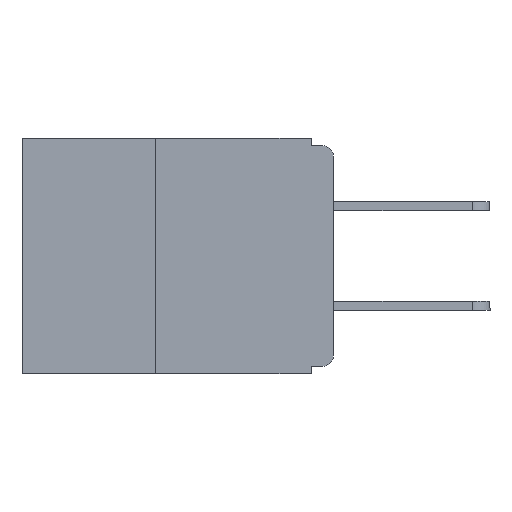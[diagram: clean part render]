
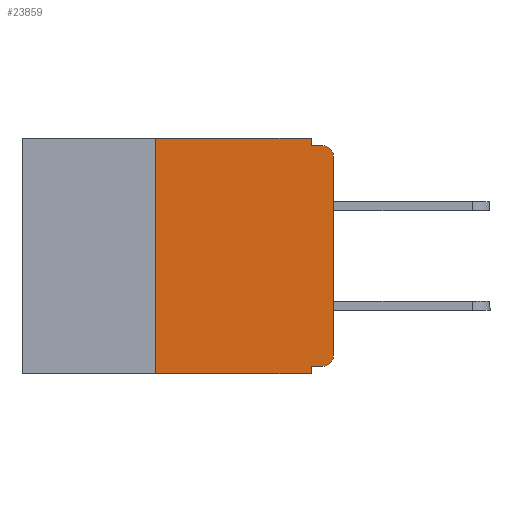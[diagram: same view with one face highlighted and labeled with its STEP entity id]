
A CAD part, left-side view. The second image highlights one B-rep face of the part: STEP entity #23859.
In plain terms, the highlighted planar face has unit normal (-1, 0, 0).
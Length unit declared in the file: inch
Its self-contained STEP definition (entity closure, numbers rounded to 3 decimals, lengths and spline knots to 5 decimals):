
#69 = EDGE_CURVE ( 'NONE', #24989, #27638, #27221, .T. ) ;
#1515 = LINE ( 'NONE', #10653, #20544 ) ;
#2247 = CARTESIAN_POINT ( 'NONE',  ( 0., 0.015, -0.32 ) ) ;
#2283 = AXIS2_PLACEMENT_3D ( 'NONE', #13039, #30058, #15529 ) ;
#2315 = CARTESIAN_POINT ( 'NONE',  ( 0., 0.015, -0.01 ) ) ;
#2810 = AXIS2_PLACEMENT_3D ( 'NONE', #7228, #9791, #26990 ) ;
#3629 = CARTESIAN_POINT ( 'NONE',  ( 0., 0., -0.32 ) ) ;
#3914 = EDGE_CURVE ( 'NONE', #24989, #8782, #6238, .T. ) ;
#5003 = DIRECTION ( 'NONE',  ( 0., 0., -1. ) ) ;
#5456 = VECTOR ( 'NONE', #20497, 39.37008 ) ;
#5634 = DIRECTION ( 'NONE',  ( 0., 0., -1. ) ) ;
#6108 = VERTEX_POINT ( 'NONE', #15819 ) ;
#6238 = LINE ( 'NONE', #23346, #5456 ) ;
#7228 = CARTESIAN_POINT ( 'NONE',  ( 0., 0.437, 0. ) ) ;
#7855 = EDGE_CURVE ( 'NONE', #8782, #6108, #23525, .T. ) ;
#8502 = VERTEX_POINT ( 'NONE', #2315 ) ;
#8549 = EDGE_CURVE ( 'NONE', #28776, #22592, #16591, .T. ) ;
#8671 = LINE ( 'NONE', #17374, #27543 ) ;
#8782 = VERTEX_POINT ( 'NONE', #28817 ) ;
#8957 = VERTEX_POINT ( 'NONE', #25981 ) ;
#9426 = ORIENTED_EDGE ( 'NONE', *, *, #69, .T. ) ;
#9603 = EDGE_CURVE ( 'NONE', #22592, #20615, #8671, .T. ) ;
#9791 = DIRECTION ( 'NONE',  ( 1., 0., 0. ) ) ;
#10653 = CARTESIAN_POINT ( 'NONE',  ( 0., 0., -0.01 ) ) ;
#11731 = CARTESIAN_POINT ( 'NONE',  ( 0., 0.25, -0.33 ) ) ;
#12016 = LINE ( 'NONE', #27891, #24304 ) ;
#13039 = CARTESIAN_POINT ( 'NONE',  ( 0., 0.015, -0.025 ) ) ;
#13706 = EDGE_LOOP ( 'NONE', ( #27013, #23572, #23749, #18823, #31264, #27578, #9426, #15834, #17494, #17732 ) ) ;
#14252 = VECTOR ( 'NONE', #24725, 39.37008 ) ;
#14523 = CARTESIAN_POINT ( 'NONE',  ( 0., 0., -0.305 ) ) ;
#15529 = DIRECTION ( 'NONE',  ( 0., 0., -1. ) ) ;
#15819 = CARTESIAN_POINT ( 'NONE',  ( 0., 0.031, 0. ) ) ;
#15834 = ORIENTED_EDGE ( 'NONE', *, *, #24614, .F. ) ;
#16591 = CIRCLE ( 'NONE', #31214, 0.015 ) ;
#16772 = DIRECTION ( 'NONE',  ( 0., 0., 1. ) ) ;
#17374 = CARTESIAN_POINT ( 'NONE',  ( 0., 0., 0. ) ) ;
#17494 = ORIENTED_EDGE ( 'NONE', *, *, #31825, .F. ) ;
#17732 = ORIENTED_EDGE ( 'NONE', *, *, #8549, .T. ) ;
#17988 = EDGE_CURVE ( 'NONE', #6108, #8957, #12016, .T. ) ;
#18161 = DIRECTION ( 'NONE',  ( 0., -1., 0. ) ) ;
#18604 = DIRECTION ( 'NONE',  ( 0., 1., 0. ) ) ;
#18823 = ORIENTED_EDGE ( 'NONE', *, *, #17988, .F. ) ;
#18871 = VECTOR ( 'NONE', #5003, 39.37008 ) ;
#20253 = CIRCLE ( 'NONE', #2283, 0.015 ) ;
#20497 = DIRECTION ( 'NONE',  ( 0., 0., 1. ) ) ;
#20544 = VECTOR ( 'NONE', #18161, 39.37008 ) ;
#20615 = VERTEX_POINT ( 'NONE', #30744 ) ;
#21401 = VERTEX_POINT ( 'NONE', #31542 ) ;
#22592 = VERTEX_POINT ( 'NONE', #14523 ) ;
#22743 = VECTOR ( 'NONE', #27589, 39.37008 ) ;
#23346 = CARTESIAN_POINT ( 'NONE',  ( 0., 0.25, -0.33 ) ) ;
#23525 = LINE ( 'NONE', #27557, #22743 ) ;
#23572 = ORIENTED_EDGE ( 'NONE', *, *, #28305, .T. ) ;
#23749 = ORIENTED_EDGE ( 'NONE', *, *, #30431, .F. ) ;
#23859 = ADVANCED_FACE ( 'NONE', ( #28788 ), #24577, .F. ) ;
#23989 = CARTESIAN_POINT ( 'NONE',  ( 0., 0.437, -0.33 ) ) ;
#24304 = VECTOR ( 'NONE', #5634, 39.37008 ) ;
#24577 = PLANE ( 'NONE',  #2810 ) ;
#24614 = EDGE_CURVE ( 'NONE', #21401, #27638, #31729, .T. ) ;
#24657 = LINE ( 'NONE', #3629, #31014 ) ;
#24725 = DIRECTION ( 'NONE',  ( 0., -1., 0. ) ) ;
#24989 = VERTEX_POINT ( 'NONE', #11731 ) ;
#25981 = CARTESIAN_POINT ( 'NONE',  ( 0., 0.031, -0.01 ) ) ;
#26990 = DIRECTION ( 'NONE',  ( 0., 0., -1. ) ) ;
#27013 = ORIENTED_EDGE ( 'NONE', *, *, #9603, .T. ) ;
#27221 = LINE ( 'NONE', #23989, #14252 ) ;
#27262 = CARTESIAN_POINT ( 'NONE',  ( 0., 0.031, -0.33 ) ) ;
#27392 = CARTESIAN_POINT ( 'NONE',  ( 0., 0.031, -0.33 ) ) ;
#27543 = VECTOR ( 'NONE', #16772, 39.37008 ) ;
#27557 = CARTESIAN_POINT ( 'NONE',  ( 0., 0.437, 0. ) ) ;
#27578 = ORIENTED_EDGE ( 'NONE', *, *, #3914, .F. ) ;
#27589 = DIRECTION ( 'NONE',  ( 0., -1., 0. ) ) ;
#27638 = VERTEX_POINT ( 'NONE', #27392 ) ;
#27891 = CARTESIAN_POINT ( 'NONE',  ( 0., 0.031, 0. ) ) ;
#28305 = EDGE_CURVE ( 'NONE', #20615, #8502, #20253, .T. ) ;
#28776 = VERTEX_POINT ( 'NONE', #2247 ) ;
#28788 = FACE_OUTER_BOUND ( 'NONE', #13706, .T. ) ;
#28817 = CARTESIAN_POINT ( 'NONE',  ( 0., 0.25, 0. ) ) ;
#30058 = DIRECTION ( 'NONE',  ( -1., 0., 0. ) ) ;
#30431 = EDGE_CURVE ( 'NONE', #8957, #8502, #1515, .T. ) ;
#30744 = CARTESIAN_POINT ( 'NONE',  ( 0., 0., -0.025 ) ) ;
#31014 = VECTOR ( 'NONE', #18604, 39.37008 ) ;
#31214 = AXIS2_PLACEMENT_3D ( 'NONE', #31839, #31776, #31733 ) ;
#31264 = ORIENTED_EDGE ( 'NONE', *, *, #7855, .F. ) ;
#31542 = CARTESIAN_POINT ( 'NONE',  ( 0., 0.031, -0.32 ) ) ;
#31729 = LINE ( 'NONE', #27262, #18871 ) ;
#31733 = DIRECTION ( 'NONE',  ( 0., 0., -1. ) ) ;
#31776 = DIRECTION ( 'NONE',  ( -1., 0., 0. ) ) ;
#31825 = EDGE_CURVE ( 'NONE', #28776, #21401, #24657, .T. ) ;
#31839 = CARTESIAN_POINT ( 'NONE',  ( 0., 0.015, -0.305 ) ) ;
